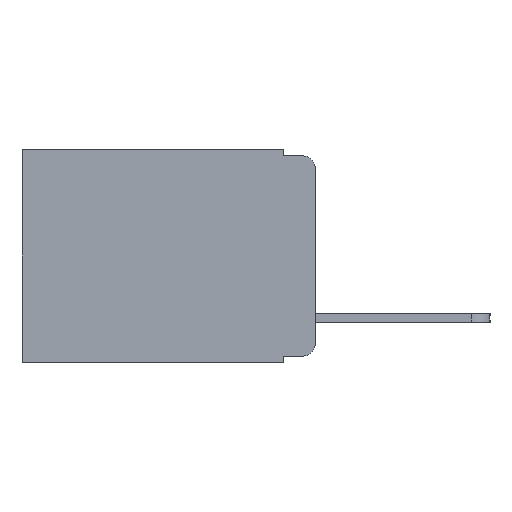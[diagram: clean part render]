
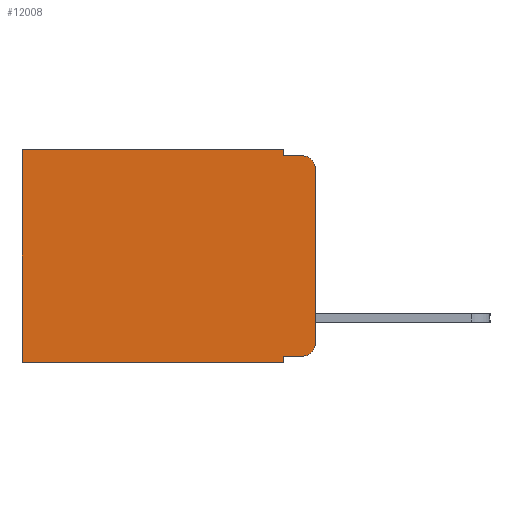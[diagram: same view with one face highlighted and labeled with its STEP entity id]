
A CAD part, left-side view. The second image highlights one B-rep face of the part: STEP entity #12008.
In plain terms, the highlighted planar face has unit normal (-1, 0, 0).
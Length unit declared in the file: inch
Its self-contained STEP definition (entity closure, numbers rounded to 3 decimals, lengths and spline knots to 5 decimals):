
#324 = DIRECTION ( 'NONE',  ( 0., 0., -1. ) ) ;
#888 = VERTEX_POINT ( 'NONE', #2118 ) ;
#1438 = LINE ( 'NONE', #13337, #11336 ) ;
#1572 = CARTESIAN_POINT ( 'NONE',  ( 0.298, 0.473, 0. ) ) ;
#2118 = CARTESIAN_POINT ( 'NONE',  ( 0.298, 0.473, -0.343 ) ) ;
#2166 = ORIENTED_EDGE ( 'NONE', *, *, #6137, .F. ) ;
#2718 = DIRECTION ( 'NONE',  ( 0., 0., -1. ) ) ;
#2947 = DIRECTION ( 'NONE',  ( 0., -1., 0. ) ) ;
#3137 = ORIENTED_EDGE ( 'NONE', *, *, #16860, .T. ) ;
#3244 = CARTESIAN_POINT ( 'NONE',  ( 0.298, 0.051, 0. ) ) ;
#3412 = CARTESIAN_POINT ( 'NONE',  ( 0.298, 0.051, 0. ) ) ;
#3569 = CARTESIAN_POINT ( 'NONE',  ( 0.298, 0., 0. ) ) ;
#3918 = LINE ( 'NONE', #9317, #14049 ) ;
#4432 = DIRECTION ( 'NONE',  ( -1., 0., 0. ) ) ;
#4583 = CARTESIAN_POINT ( 'NONE',  ( 0.298, 0.051, -0.333 ) ) ;
#4931 = VERTEX_POINT ( 'NONE', #15778 ) ;
#5070 = ORIENTED_EDGE ( 'NONE', *, *, #15830, .T. ) ;
#5327 = CARTESIAN_POINT ( 'NONE',  ( 0.298, 0., 0. ) ) ;
#6019 = EDGE_LOOP ( 'NONE', ( #2166, #12423, #16729, #10633, #5070, #3137, #17046, #15640, #11732, #13833 ) ) ;
#6137 = EDGE_CURVE ( 'NONE', #12820, #4931, #3918, .T. ) ;
#6351 = LINE ( 'NONE', #3569, #12965 ) ;
#6443 = CARTESIAN_POINT ( 'NONE',  ( 0.298, 0.051, -0.333 ) ) ;
#6703 = DIRECTION ( 'NONE',  ( 1., 0., 0. ) ) ;
#6915 = LINE ( 'NONE', #10962, #10048 ) ;
#7184 = EDGE_CURVE ( 'NONE', #9959, #14387, #15340, .T. ) ;
#7640 = DIRECTION ( 'NONE',  ( 0., 1., 0. ) ) ;
#7772 = CARTESIAN_POINT ( 'NONE',  ( 0.298, 0.051, -0.343 ) ) ;
#8123 = CARTESIAN_POINT ( 'NONE',  ( 0.298, 0.051, -0.01 ) ) ;
#8489 = DIRECTION ( 'NONE',  ( -1., 0., 0. ) ) ;
#8526 = CARTESIAN_POINT ( 'NONE',  ( 0.298, 0.473, 0. ) ) ;
#8578 = VERTEX_POINT ( 'NONE', #7772 ) ;
#8729 = EDGE_CURVE ( 'NONE', #11929, #16711, #15475, .T. ) ;
#8841 = EDGE_CURVE ( 'NONE', #14387, #4931, #10530, .T. ) ;
#9128 = LINE ( 'NONE', #3244, #12588 ) ;
#9256 = DIRECTION ( 'NONE',  ( 0., 0., -1. ) ) ;
#9271 = CIRCLE ( 'NONE', #11271, 0.02 ) ;
#9317 = CARTESIAN_POINT ( 'NONE',  ( 0.298, 0., 0. ) ) ;
#9357 = VECTOR ( 'NONE', #13464, 39.37008 ) ;
#9419 = EDGE_CURVE ( 'NONE', #12820, #13626, #9271, .T. ) ;
#9959 = VERTEX_POINT ( 'NONE', #4583 ) ;
#10048 = VECTOR ( 'NONE', #2947, 39.37008 ) ;
#10155 = DIRECTION ( 'NONE',  ( 0., 0., -1. ) ) ;
#10530 = CIRCLE ( 'NONE', #15282, 0.02 ) ;
#10633 = ORIENTED_EDGE ( 'NONE', *, *, #8729, .F. ) ;
#10962 = CARTESIAN_POINT ( 'NONE',  ( 0.298, 0.051, -0.01 ) ) ;
#11100 = AXIS2_PLACEMENT_3D ( 'NONE', #5327, #6703, #15744 ) ;
#11243 = DIRECTION ( 'NONE',  ( 0., 0., -1. ) ) ;
#11245 = CARTESIAN_POINT ( 'NONE',  ( 0.298, 0.02, -0.333 ) ) ;
#11271 = AXIS2_PLACEMENT_3D ( 'NONE', #16143, #8489, #9256 ) ;
#11302 = LINE ( 'NONE', #8526, #14697 ) ;
#11336 = VECTOR ( 'NONE', #12054, 39.37008 ) ;
#11732 = ORIENTED_EDGE ( 'NONE', *, *, #7184, .T. ) ;
#11747 = CARTESIAN_POINT ( 'NONE',  ( 0.298, 0., -0.03 ) ) ;
#11929 = VERTEX_POINT ( 'NONE', #15584 ) ;
#12008 = ADVANCED_FACE ( 'NONE', ( #12086 ), #13260, .F. ) ;
#12054 = DIRECTION ( 'NONE',  ( 0., 1., 0. ) ) ;
#12086 = FACE_OUTER_BOUND ( 'NONE', #6019, .T. ) ;
#12143 = EDGE_CURVE ( 'NONE', #16711, #13626, #6915, .T. ) ;
#12146 = VECTOR ( 'NONE', #10155, 39.37008 ) ;
#12406 = CARTESIAN_POINT ( 'NONE',  ( 0.298, 0.02, -0.313 ) ) ;
#12423 = ORIENTED_EDGE ( 'NONE', *, *, #9419, .T. ) ;
#12588 = VECTOR ( 'NONE', #11243, 39.37008 ) ;
#12820 = VERTEX_POINT ( 'NONE', #11747 ) ;
#12965 = VECTOR ( 'NONE', #7640, 39.37008 ) ;
#13260 = PLANE ( 'NONE',  #11100 ) ;
#13337 = CARTESIAN_POINT ( 'NONE',  ( 0.298, 0., -0.343 ) ) ;
#13464 = DIRECTION ( 'NONE',  ( 0., -1., 0. ) ) ;
#13626 = VERTEX_POINT ( 'NONE', #17139 ) ;
#13696 = DIRECTION ( 'NONE',  ( 0., 0., -1. ) ) ;
#13833 = ORIENTED_EDGE ( 'NONE', *, *, #8841, .T. ) ;
#14049 = VECTOR ( 'NONE', #2718, 39.37008 ) ;
#14387 = VERTEX_POINT ( 'NONE', #11245 ) ;
#14697 = VECTOR ( 'NONE', #324, 39.37008 ) ;
#14896 = VERTEX_POINT ( 'NONE', #1572 ) ;
#15080 = EDGE_CURVE ( 'NONE', #9959, #8578, #9128, .T. ) ;
#15282 = AXIS2_PLACEMENT_3D ( 'NONE', #12406, #4432, #13696 ) ;
#15340 = LINE ( 'NONE', #6443, #9357 ) ;
#15475 = LINE ( 'NONE', #3412, #12146 ) ;
#15584 = CARTESIAN_POINT ( 'NONE',  ( 0.298, 0.051, 0. ) ) ;
#15640 = ORIENTED_EDGE ( 'NONE', *, *, #15080, .F. ) ;
#15744 = DIRECTION ( 'NONE',  ( 0., 0., -1. ) ) ;
#15778 = CARTESIAN_POINT ( 'NONE',  ( 0.298, 0., -0.313 ) ) ;
#15830 = EDGE_CURVE ( 'NONE', #11929, #14896, #6351, .T. ) ;
#16072 = EDGE_CURVE ( 'NONE', #8578, #888, #1438, .T. ) ;
#16143 = CARTESIAN_POINT ( 'NONE',  ( 0.298, 0.02, -0.03 ) ) ;
#16711 = VERTEX_POINT ( 'NONE', #8123 ) ;
#16729 = ORIENTED_EDGE ( 'NONE', *, *, #12143, .F. ) ;
#16860 = EDGE_CURVE ( 'NONE', #14896, #888, #11302, .T. ) ;
#17046 = ORIENTED_EDGE ( 'NONE', *, *, #16072, .F. ) ;
#17139 = CARTESIAN_POINT ( 'NONE',  ( 0.298, 0.02, -0.01 ) ) ;
